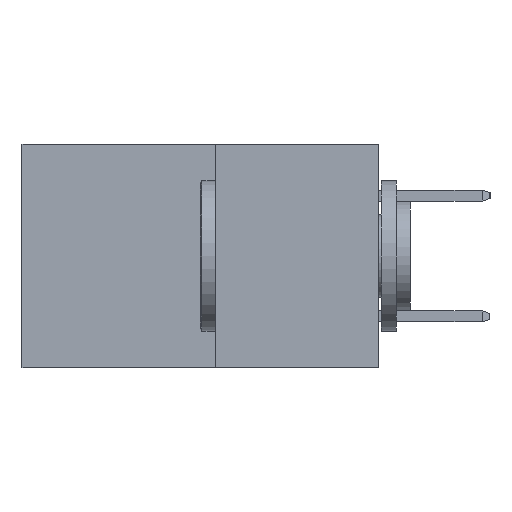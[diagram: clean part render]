
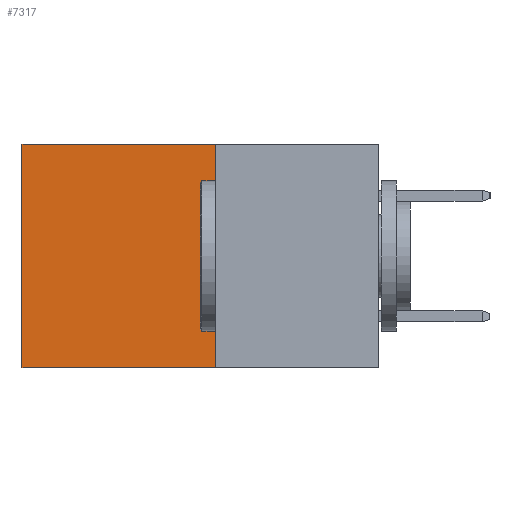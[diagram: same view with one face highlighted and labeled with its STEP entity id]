
A CAD part, left-side view. The second image highlights one B-rep face of the part: STEP entity #7317.
In plain terms, the highlighted planar face has unit normal (-1, 0, 0).
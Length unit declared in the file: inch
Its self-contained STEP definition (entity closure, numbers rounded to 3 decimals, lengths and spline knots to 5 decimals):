
#692 = LINE ( 'NONE', #11705, #4157 ) ;
#1125 = AXIS2_PLACEMENT_3D ( 'NONE', #6169, #1603, #9621 ) ;
#1313 = EDGE_CURVE ( 'NONE', #8264, #11383, #14688, .T. ) ;
#1335 = VERTEX_POINT ( 'NONE', #2295 ) ;
#1603 = DIRECTION ( 'NONE',  ( 1., 0., 0. ) ) ;
#1787 = EDGE_LOOP ( 'NONE', ( #12007, #12224, #4287, #3570 ) ) ;
#1815 = LINE ( 'NONE', #11451, #13632 ) ;
#2081 = CARTESIAN_POINT ( 'NONE',  ( 0.277, 0.27, -0.37 ) ) ;
#2295 = CARTESIAN_POINT ( 'NONE',  ( 0.277, 0.59, 0. ) ) ;
#2969 = CARTESIAN_POINT ( 'NONE',  ( 0.277, 0.27, -0.37 ) ) ;
#3570 = ORIENTED_EDGE ( 'NONE', *, *, #7679, .T. ) ;
#3755 = DIRECTION ( 'NONE',  ( 0., 0., -1. ) ) ;
#4157 = VECTOR ( 'NONE', #3755, 39.37008 ) ;
#4287 = ORIENTED_EDGE ( 'NONE', *, *, #11674, .F. ) ;
#4772 = VECTOR ( 'NONE', #9348, 39.37008 ) ;
#5062 = PLANE ( 'NONE',  #1125 ) ;
#6124 = FACE_OUTER_BOUND ( 'NONE', #1787, .T. ) ;
#6169 = CARTESIAN_POINT ( 'NONE',  ( 0.277, 0.27, -0.37 ) ) ;
#6908 = DIRECTION ( 'NONE',  ( 0., 1., 0. ) ) ;
#7317 = ADVANCED_FACE ( 'NONE', ( #6124 ), #5062, .F. ) ;
#7375 = VERTEX_POINT ( 'NONE', #9833 ) ;
#7679 = EDGE_CURVE ( 'NONE', #7375, #1335, #1815, .T. ) ;
#8056 = DIRECTION ( 'NONE',  ( 0., 1., 0. ) ) ;
#8264 = VERTEX_POINT ( 'NONE', #2081 ) ;
#9107 = EDGE_CURVE ( 'NONE', #1335, #11383, #692, .T. ) ;
#9348 = DIRECTION ( 'NONE',  ( 0., 0., -1. ) ) ;
#9621 = DIRECTION ( 'NONE',  ( 0., 0., -1. ) ) ;
#9833 = CARTESIAN_POINT ( 'NONE',  ( 0.277, 0.27, 0. ) ) ;
#10434 = CARTESIAN_POINT ( 'NONE',  ( 0.277, 0.27, -0.37 ) ) ;
#10797 = LINE ( 'NONE', #10434, #4772 ) ;
#11383 = VERTEX_POINT ( 'NONE', #14542 ) ;
#11451 = CARTESIAN_POINT ( 'NONE',  ( 0.277, 0.27, 0. ) ) ;
#11664 = VECTOR ( 'NONE', #6908, 39.37008 ) ;
#11674 = EDGE_CURVE ( 'NONE', #7375, #8264, #10797, .T. ) ;
#11705 = CARTESIAN_POINT ( 'NONE',  ( 0.277, 0.59, -0.37 ) ) ;
#12007 = ORIENTED_EDGE ( 'NONE', *, *, #9107, .T. ) ;
#12224 = ORIENTED_EDGE ( 'NONE', *, *, #1313, .F. ) ;
#13632 = VECTOR ( 'NONE', #8056, 39.37008 ) ;
#14542 = CARTESIAN_POINT ( 'NONE',  ( 0.277, 0.59, -0.37 ) ) ;
#14688 = LINE ( 'NONE', #2969, #11664 ) ;
